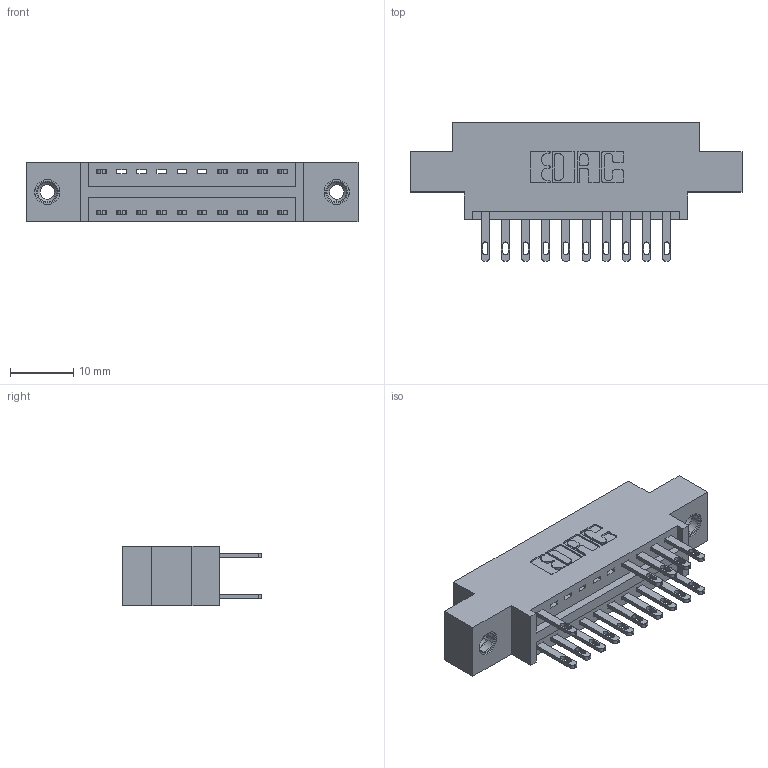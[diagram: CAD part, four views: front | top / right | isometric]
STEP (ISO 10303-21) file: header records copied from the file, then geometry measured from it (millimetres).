
FILE_DESCRIPTION (( 'STEP AP203' ), '1' );
FILE_NAME ('346-020-500-808.STEP', '2018-08-20T10:54:48', ( '' ), ( '' ), 'SwSTEP 2.0', 'SolidWorks 2016', '' );
FILE_SCHEMA (( 'CONFIG_CONTROL_DESIGN' ));
Length unit declared in the file: inch
Products named in the file (4): 346 Part_0.170 Offset - 0.156 Dia-TI; 345-292-001_345-293-100; 345-250-001_345-250-003-102; 346-020-500-808
Assembly tree (18 placements, depth 2):
  346-020-500-808
    346 Part_0.170 Offset - 0.156 Dia-TI
    345-292-001_345-293-100  x15
    345-250-001_345-250-003-102  x2
Bounding box: 52.32 x 21.84 x 9.4 mm (x, y, z)
Volume: 4693.4 mm3; surface area: 6045.6 mm2
Topology: 18 solids, 18 shells, 936 faces, 2787 edges, 1850 vertices
Faces by surface type: plane 572, cylinder 348, cone 12, torus 4
Entity records: 11922 total; most frequent: CARTESIAN_POINT 2014, ORIENTED_EDGE 1946, DIRECTION 1849, EDGE_CURVE 973, VECTOR 777, LINE 777, VERTEX_POINT 644, AXIS2_PLACEMENT_3D 536
